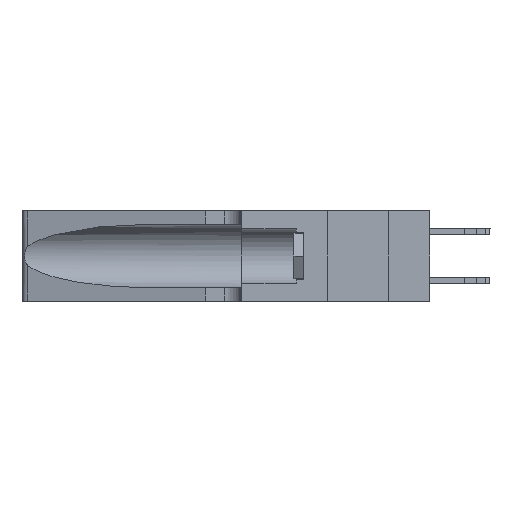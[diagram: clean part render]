
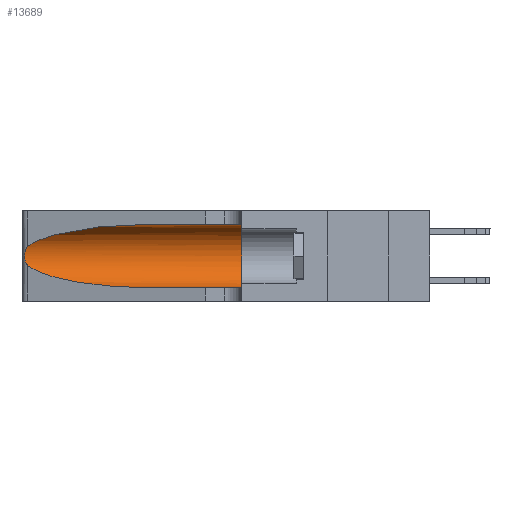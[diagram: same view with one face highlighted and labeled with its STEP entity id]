
A CAD part, left-side view. The second image highlights one B-rep face of the part: STEP entity #13689.
In plain terms, the highlighted cylindrical face has radius 3.308 mm (diameter 6.617 mm), a partial arc.
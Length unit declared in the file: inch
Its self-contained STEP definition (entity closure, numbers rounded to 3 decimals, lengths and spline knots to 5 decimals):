
#87 = LINE ( 'NONE', #7921, #1373 ) ;
#989 = CARTESIAN_POINT ( 'NONE',  ( 0.26075, 1.23896, 0.178 ) ) ;
#1100 = CARTESIAN_POINT ( 'NONE',  ( 0.25789, 1.23486, 0.15765 ) ) ;
#1373 = VECTOR ( 'NONE', #30094, 39.37008 ) ;
#1957 = ORIENTED_EDGE ( 'NONE', *, *, #28136, .T. ) ;
#2889 = CARTESIAN_POINT ( 'NONE',  ( 0.18966, 0.96281, 0.31525 ) ) ;
#3178 = ORIENTED_EDGE ( 'NONE', *, *, #35220, .T. ) ;
#3185 = EDGE_LOOP ( 'NONE', ( #34387, #1957, #7175, #3178, #25328, #20852 ) ) ;
#3475 = VERTEX_POINT ( 'NONE', #11107 ) ;
#3767 = CARTESIAN_POINT ( 'NONE',  ( 0.26017, 1.23833, 0.17102 ) ) ;
#4086 =( BOUNDED_CURVE ( )  B_SPLINE_CURVE ( 3, ( #29690, #26772, #24385, #7532 ),
 .UNSPECIFIED., .F., .T. ) 
 B_SPLINE_CURVE_WITH_KNOTS ( ( 4, 4 ),
 ( 3.44316, 4.71239 ),
 .UNSPECIFIED. ) 
 CURVE ( )  GEOMETRIC_REPRESENTATION_ITEM ( )  RATIONAL_B_SPLINE_CURVE ( ( 1., 0.87, 0.87, 1. ) ) 
 REPRESENTATION_ITEM ( '' )  );
#4220 = DIRECTION ( 'NONE',  ( 0., -1., 0. ) ) ;
#5197 = B_SPLINE_CURVE_WITH_KNOTS ( 'NONE', 3,
 ( #15205, #34381, #34270, #23486, #12440, #17519, #12208, #989, #3767, #17652, #1100, #10232, #26695, #18363 ),
 .UNSPECIFIED., .F., .F.,
 ( 4, 2, 2, 2, 2, 2, 4 ),
 ( 0., 0.00027, 0.00053, 0.00107, 0.0016, 0.00187, 0.00214 ),
 .UNSPECIFIED. ) ;
#5452 = CARTESIAN_POINT ( 'NONE',  ( 0.25487, 1.22718, 0.14631 ) ) ;
#5854 = CARTESIAN_POINT ( 'NONE',  ( 0.25487, 1.22718, 0.22369 ) ) ;
#6501 = VERTEX_POINT ( 'NONE', #28824 ) ;
#7175 = ORIENTED_EDGE ( 'NONE', *, *, #29524, .T. ) ;
#7532 = CARTESIAN_POINT ( 'NONE',  ( 0.1305, 0.72297, 0.05475 ) ) ;
#7921 = CARTESIAN_POINT ( 'NONE',  ( 0.1305, 1.61858, 0.05475 ) ) ;
#10033 = DIRECTION ( 'NONE',  ( 0., 0., -1. ) ) ;
#10232 = CARTESIAN_POINT ( 'NONE',  ( 0.25639, 1.23186, 0.15144 ) ) ;
#11107 = CARTESIAN_POINT ( 'NONE',  ( 0.1305, 0.35, 0.31525 ) ) ;
#11188 = CARTESIAN_POINT ( 'NONE',  ( 0.1305, 0.72297, 0.31525 ) ) ;
#11222 = CARTESIAN_POINT ( 'NONE',  ( 0.1305, 0.35, 0.185 ) ) ;
#12186 = CYLINDRICAL_SURFACE ( 'NONE', #15270, 0.13025 ) ;
#12208 = CARTESIAN_POINT ( 'NONE',  ( 0.26075, 1.23896, 0.19203 ) ) ;
#12440 = CARTESIAN_POINT ( 'NONE',  ( 0.25854, 1.2359, 0.20912 ) ) ;
#13236 = LINE ( 'NONE', #35215, #22813 ) ;
#13689 = ADVANCED_FACE ( 'NONE', ( #31716 ), #12186, .F. ) ;
#15205 = CARTESIAN_POINT ( 'NONE',  ( 0.25487, 1.22718, 0.22369 ) ) ;
#15270 = AXIS2_PLACEMENT_3D ( 'NONE', #15345, #32095, #10033 ) ;
#15345 = CARTESIAN_POINT ( 'NONE',  ( 0.1305, 1.61858, 0.185 ) ) ;
#15490 = VERTEX_POINT ( 'NONE', #11188 ) ;
#15608 = CARTESIAN_POINT ( 'NONE',  ( 0.1305, 0.72297, 0.05475 ) ) ;
#17172 = AXIS2_PLACEMENT_3D ( 'NONE', #11222, #22376, #28034 ) ;
#17519 = CARTESIAN_POINT ( 'NONE',  ( 0.26018, 1.23835, 0.19895 ) ) ;
#17652 = CARTESIAN_POINT ( 'NONE',  ( 0.25856, 1.23593, 0.16098 ) ) ;
#18363 = CARTESIAN_POINT ( 'NONE',  ( 0.25487, 1.22718, 0.14631 ) ) ;
#18953 = VERTEX_POINT ( 'NONE', #33515 ) ;
#20290 =( BOUNDED_CURVE ( )  B_SPLINE_CURVE ( 3, ( #22354, #2889, #25333, #5854 ),
 .UNSPECIFIED., .F., .F. ) 
 B_SPLINE_CURVE_WITH_KNOTS ( ( 4, 4 ),
 ( 1.5708, 2.84003 ),
 .UNSPECIFIED. ) 
 CURVE ( )  GEOMETRIC_REPRESENTATION_ITEM ( )  RATIONAL_B_SPLINE_CURVE ( ( 1., 0.87, 0.87, 1. ) ) 
 REPRESENTATION_ITEM ( '' )  );
#20852 = ORIENTED_EDGE ( 'NONE', *, *, #28279, .F. ) ;
#22354 = CARTESIAN_POINT ( 'NONE',  ( 0.1305, 0.72297, 0.31525 ) ) ;
#22376 = DIRECTION ( 'NONE',  ( 0., 1., 0. ) ) ;
#22813 = VECTOR ( 'NONE', #4220, 39.37008 ) ;
#23486 = CARTESIAN_POINT ( 'NONE',  ( 0.25787, 1.23484, 0.2124 ) ) ;
#24112 = VERTEX_POINT ( 'NONE', #5452 ) ;
#24385 = CARTESIAN_POINT ( 'NONE',  ( 0.18966, 0.96281, 0.05475 ) ) ;
#25328 = ORIENTED_EDGE ( 'NONE', *, *, #28610, .F. ) ;
#25333 = CARTESIAN_POINT ( 'NONE',  ( 0.2373, 1.15595, 0.28018 ) ) ;
#25352 = CIRCLE ( 'NONE', #17172, 0.13025 ) ;
#26695 = CARTESIAN_POINT ( 'NONE',  ( 0.25555, 1.22993, 0.14849 ) ) ;
#26772 = CARTESIAN_POINT ( 'NONE',  ( 0.2373, 1.15595, 0.08982 ) ) ;
#27551 = VERTEX_POINT ( 'NONE', #15608 ) ;
#28034 = DIRECTION ( 'NONE',  ( 0., 0., 1. ) ) ;
#28136 = EDGE_CURVE ( 'NONE', #6501, #24112, #5197, .T. ) ;
#28279 = EDGE_CURVE ( 'NONE', #15490, #3475, #13236, .T. ) ;
#28610 = EDGE_CURVE ( 'NONE', #3475, #18953, #25352, .T. ) ;
#28824 = CARTESIAN_POINT ( 'NONE',  ( 0.25487, 1.22718, 0.22369 ) ) ;
#29524 = EDGE_CURVE ( 'NONE', #24112, #27551, #4086, .T. ) ;
#29690 = CARTESIAN_POINT ( 'NONE',  ( 0.25487, 1.22718, 0.14631 ) ) ;
#30094 = DIRECTION ( 'NONE',  ( 0., -1., 0. ) ) ;
#31716 = FACE_OUTER_BOUND ( 'NONE', #3185, .T. ) ;
#32095 = DIRECTION ( 'NONE',  ( 0., -1., 0. ) ) ;
#33515 = CARTESIAN_POINT ( 'NONE',  ( 0.1305, 0.35, 0.05475 ) ) ;
#33800 = EDGE_CURVE ( 'NONE', #15490, #6501, #20290, .T. ) ;
#34270 = CARTESIAN_POINT ( 'NONE',  ( 0.25639, 1.23184, 0.21858 ) ) ;
#34381 = CARTESIAN_POINT ( 'NONE',  ( 0.25555, 1.22994, 0.2215 ) ) ;
#34387 = ORIENTED_EDGE ( 'NONE', *, *, #33800, .T. ) ;
#35215 = CARTESIAN_POINT ( 'NONE',  ( 0.1305, 1.61858, 0.31525 ) ) ;
#35220 = EDGE_CURVE ( 'NONE', #27551, #18953, #87, .T. ) ;
